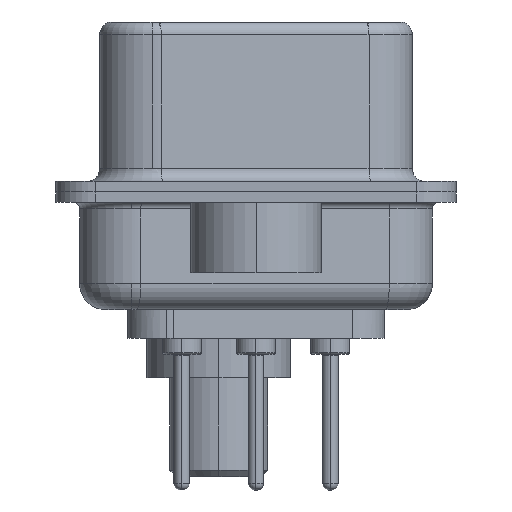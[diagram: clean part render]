
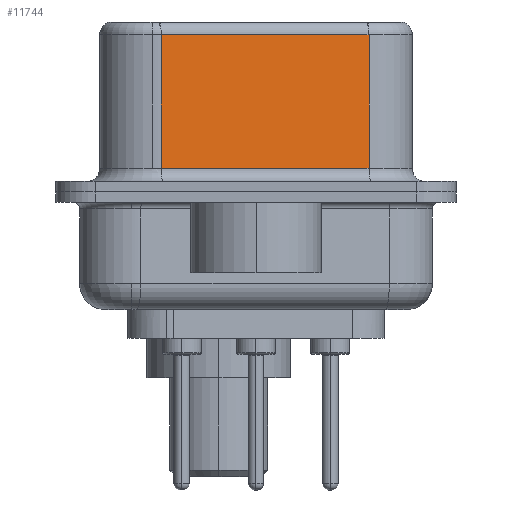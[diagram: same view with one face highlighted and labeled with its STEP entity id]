
A CAD part, left-side view. The second image highlights one B-rep face of the part: STEP entity #11744.
In plain terms, the highlighted planar face has unit normal (-0.985, -0.174, 0).
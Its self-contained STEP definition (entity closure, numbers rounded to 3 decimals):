
#399 = LINE ( 'NONE', #19174, #5622 ) ;
#863 = PLANE ( 'NONE',  #16471 ) ;
#2109 = VECTOR ( 'NONE', #13035, 1000. ) ;
#2923 = EDGE_CURVE ( 'NONE', #27684, #27111, #20731, .T. ) ;
#3119 = VECTOR ( 'NONE', #6328, 1000. ) ;
#3299 = EDGE_LOOP ( 'NONE', ( #10337, #23804, #20718, #18095 ) ) ;
#4083 = DIRECTION ( 'NONE',  ( -0.174, 0.985, 0. ) ) ;
#5622 = VECTOR ( 'NONE', #16956, 1000. ) ;
#6328 = DIRECTION ( 'NONE',  ( 0., 0., -1. ) ) ;
#7056 = VECTOR ( 'NONE', #4083, 1000. ) ;
#7354 = EDGE_CURVE ( 'NONE', #25484, #27111, #399, .T. ) ;
#7576 = CARTESIAN_POINT ( 'NONE',  ( 5.132, -4.322, 6.52 ) ) ;
#7751 = LINE ( 'NONE', #28272, #7056 ) ;
#9423 = EDGE_CURVE ( 'NONE', #12649, #25484, #19752, .T. ) ;
#9795 = DIRECTION ( 'NONE',  ( -0.174, 0.985, 0. ) ) ;
#10337 = ORIENTED_EDGE ( 'NONE', *, *, #2923, .F. ) ;
#10914 = CARTESIAN_POINT ( 'NONE',  ( 3.73, 3.628, 6.02 ) ) ;
#11744 = ADVANCED_FACE ( 'NONE', ( #11897 ), #863, .F. ) ;
#11897 = FACE_OUTER_BOUND ( 'NONE', #3299, .T. ) ;
#11997 = EDGE_CURVE ( 'NONE', #27684, #12649, #7751, .T. ) ;
#12649 = VERTEX_POINT ( 'NONE', #10914 ) ;
#13035 = DIRECTION ( 'NONE',  ( 0., 0., -1. ) ) ;
#15291 = CARTESIAN_POINT ( 'NONE',  ( 3.73, 3.628, 6.52 ) ) ;
#16337 = CARTESIAN_POINT ( 'NONE',  ( 5.132, -4.322, 6.52 ) ) ;
#16471 = AXIS2_PLACEMENT_3D ( 'NONE', #7576, #23025, #9795 ) ;
#16956 = DIRECTION ( 'NONE',  ( 0.174, -0.985, 0. ) ) ;
#17659 = CARTESIAN_POINT ( 'NONE',  ( 5.132, -4.322, 6.02 ) ) ;
#18095 = ORIENTED_EDGE ( 'NONE', *, *, #7354, .T. ) ;
#19174 = CARTESIAN_POINT ( 'NONE',  ( 5.132, -4.322, 0.9 ) ) ;
#19752 = LINE ( 'NONE', #15291, #2109 ) ;
#20234 = CARTESIAN_POINT ( 'NONE',  ( 3.73, 3.628, 0.9 ) ) ;
#20718 = ORIENTED_EDGE ( 'NONE', *, *, #9423, .T. ) ;
#20731 = LINE ( 'NONE', #16337, #3119 ) ;
#23025 = DIRECTION ( 'NONE',  ( 0.985, 0.174, 0. ) ) ;
#23804 = ORIENTED_EDGE ( 'NONE', *, *, #11997, .T. ) ;
#24747 = CARTESIAN_POINT ( 'NONE',  ( 5.132, -4.322, 0.9 ) ) ;
#25484 = VERTEX_POINT ( 'NONE', #20234 ) ;
#27111 = VERTEX_POINT ( 'NONE', #24747 ) ;
#27684 = VERTEX_POINT ( 'NONE', #17659 ) ;
#28272 = CARTESIAN_POINT ( 'NONE',  ( 5.132, -4.322, 6.02 ) ) ;
